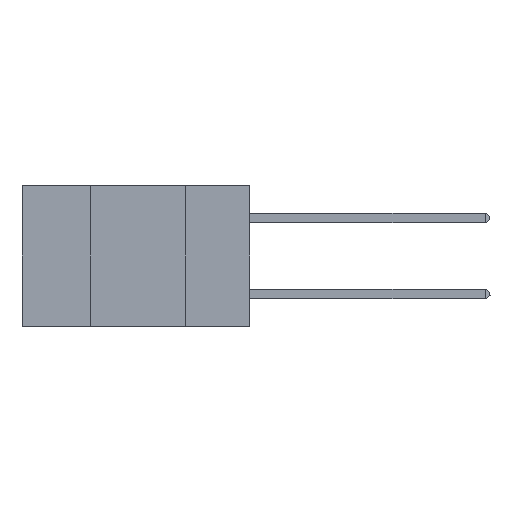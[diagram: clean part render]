
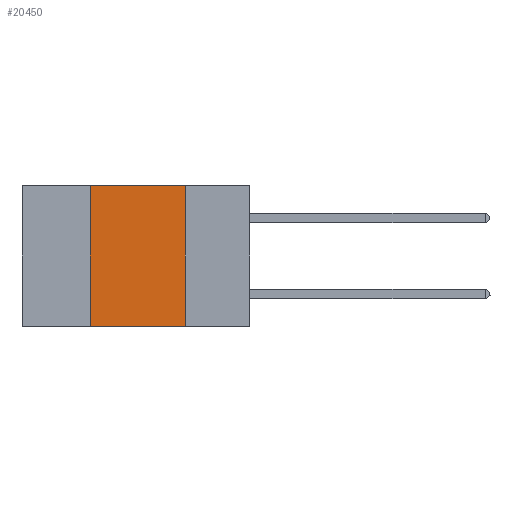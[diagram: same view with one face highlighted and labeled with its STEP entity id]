
A CAD part, left-side view. The second image highlights one B-rep face of the part: STEP entity #20450.
In plain terms, the highlighted planar face has unit normal (-1, 0, 0).
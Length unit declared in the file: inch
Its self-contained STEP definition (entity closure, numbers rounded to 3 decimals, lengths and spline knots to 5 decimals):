
#2330 = VERTEX_POINT ( 'NONE', #30034 ) ;
#3322 = ORIENTED_EDGE ( 'NONE', *, *, #18536, .F. ) ;
#4196 = CARTESIAN_POINT ( 'NONE',  ( 0., 0.6, 0. ) ) ;
#4811 = LINE ( 'NONE', #20714, #19279 ) ;
#4868 = FACE_OUTER_BOUND ( 'NONE', #23702, .T. ) ;
#9327 = DIRECTION ( 'NONE',  ( 0., -1., 0. ) ) ;
#9568 = ORIENTED_EDGE ( 'NONE', *, *, #35267, .T. ) ;
#12045 = DIRECTION ( 'NONE',  ( 0., 0., 1. ) ) ;
#13229 = CARTESIAN_POINT ( 'NONE',  ( 0., 0.42, 0. ) ) ;
#14560 = AXIS2_PLACEMENT_3D ( 'NONE', #4196, #23718, #26742 ) ;
#18231 = VERTEX_POINT ( 'NONE', #13229 ) ;
#18536 = EDGE_CURVE ( 'NONE', #2330, #18231, #27816, .T. ) ;
#19279 = VECTOR ( 'NONE', #29598, 39.37008 ) ;
#19488 = CARTESIAN_POINT ( 'NONE',  ( 0., 0.17, -0.37 ) ) ;
#20450 = ADVANCED_FACE ( 'NONE', ( #4868 ), #31941, .F. ) ;
#20714 = CARTESIAN_POINT ( 'NONE',  ( 0., 0.6, -0.37 ) ) ;
#21021 = DIRECTION ( 'NONE',  ( 0., 0., -1. ) ) ;
#21152 = VECTOR ( 'NONE', #9327, 39.37008 ) ;
#23066 = CARTESIAN_POINT ( 'NONE',  ( 0., 0.17, 0. ) ) ;
#23185 = VERTEX_POINT ( 'NONE', #19488 ) ;
#23702 = EDGE_LOOP ( 'NONE', ( #35675, #30201, #3322, #9568 ) ) ;
#23718 = DIRECTION ( 'NONE',  ( 1., 0., 0. ) ) ;
#24105 = CARTESIAN_POINT ( 'NONE',  ( 0., 0.17, 0. ) ) ;
#25715 = LINE ( 'NONE', #24105, #28378 ) ;
#26742 = DIRECTION ( 'NONE',  ( 0., 0., -1. ) ) ;
#27816 = LINE ( 'NONE', #28585, #36218 ) ;
#28378 = VECTOR ( 'NONE', #21021, 39.37008 ) ;
#28585 = CARTESIAN_POINT ( 'NONE',  ( 0., 0.42, 0. ) ) ;
#28939 = CARTESIAN_POINT ( 'NONE',  ( 0., 0.6, 0. ) ) ;
#29598 = DIRECTION ( 'NONE',  ( 0., -1., 0. ) ) ;
#30034 = CARTESIAN_POINT ( 'NONE',  ( 0., 0.42, -0.37 ) ) ;
#30201 = ORIENTED_EDGE ( 'NONE', *, *, #33827, .F. ) ;
#30763 = EDGE_CURVE ( 'NONE', #35108, #23185, #25715, .T. ) ;
#31941 = PLANE ( 'NONE',  #14560 ) ;
#32621 = LINE ( 'NONE', #28939, #21152 ) ;
#33827 = EDGE_CURVE ( 'NONE', #18231, #35108, #32621, .T. ) ;
#35108 = VERTEX_POINT ( 'NONE', #23066 ) ;
#35267 = EDGE_CURVE ( 'NONE', #2330, #23185, #4811, .T. ) ;
#35675 = ORIENTED_EDGE ( 'NONE', *, *, #30763, .F. ) ;
#36218 = VECTOR ( 'NONE', #12045, 39.37008 ) ;
